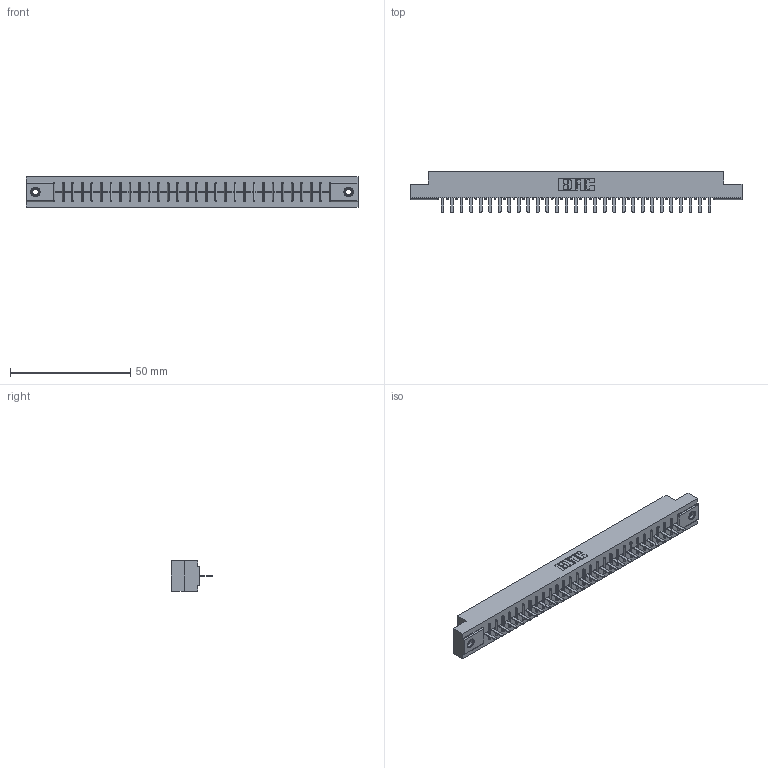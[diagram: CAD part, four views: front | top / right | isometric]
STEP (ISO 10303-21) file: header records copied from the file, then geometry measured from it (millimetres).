
FILE_DESCRIPTION (( 'STEP AP203' ), '1' );
FILE_NAME ('306-029-520-107.STEP', '2019-09-11T22:11:24', ( '' ), ( '' ), 'SwSTEP 2.0', 'SolidWorks 2016', '' );
FILE_SCHEMA (( 'CONFIG_CONTROL_DESIGN' ));
Length unit declared in the file: inch
Products named in the file (4): 306-290-001_120; 306-029-520-107; 306 Part_.156 Dia; 345-250-001_345-250-005-103
Assembly tree (32 placements, depth 2):
  306-029-520-107
    306 Part_.156 Dia
    306-290-001_120  x29
    345-250-001_345-250-005-103  x2
Bounding box: 137.92 x 17.12 x 12.7 mm (x, y, z)
Volume: 15121.5 mm3; surface area: 15431.7 mm2
Topology: 32 solids, 32 shells, 2206 faces, 6165 edges, 3946 vertices
Faces by surface type: plane 1463, cylinder 611, sphere 116, cone 12, torus 4
Entity records: 29869 total; most frequent: CARTESIAN_POINT 4993, ORIENTED_EDGE 4942, DIRECTION 4933, EDGE_CURVE 2471, VECTOR 1925, LINE 1925, VERTEX_POINT 1564, AXIS2_PLACEMENT_3D 1504
